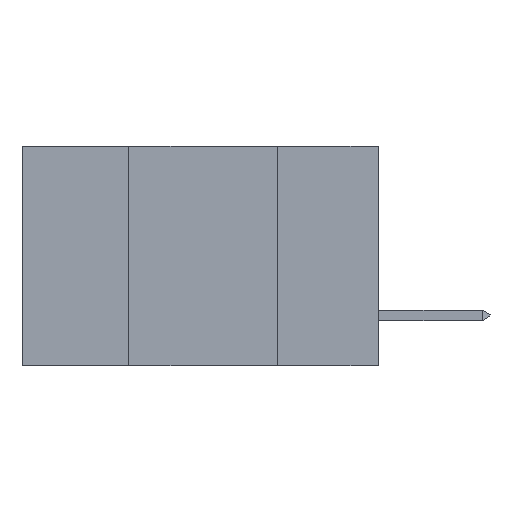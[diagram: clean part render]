
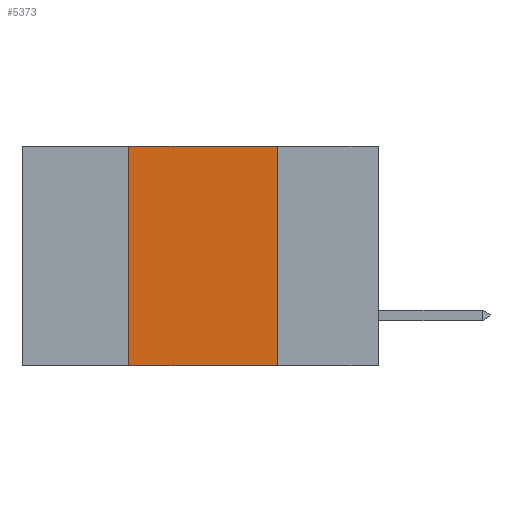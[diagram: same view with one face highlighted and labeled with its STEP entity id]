
A CAD part, left-side view. The second image highlights one B-rep face of the part: STEP entity #5373.
In plain terms, the highlighted planar face has unit normal (-1, 0, 0).
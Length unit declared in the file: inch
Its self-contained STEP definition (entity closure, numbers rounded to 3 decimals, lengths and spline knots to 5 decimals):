
#425 = VERTEX_POINT ( 'NONE', #5823 ) ;
#1154 = CARTESIAN_POINT ( 'NONE',  ( 0., 0.17, -0.37 ) ) ;
#1305 = FACE_OUTER_BOUND ( 'NONE', #10136, .T. ) ;
#1309 = LINE ( 'NONE', #15162, #5627 ) ;
#2109 = CARTESIAN_POINT ( 'NONE',  ( 0., 0.42, 0. ) ) ;
#2255 = EDGE_CURVE ( 'NONE', #4426, #10716, #3653, .T. ) ;
#2405 = CARTESIAN_POINT ( 'NONE',  ( 0., 0.6, -0.37 ) ) ;
#2849 = ORIENTED_EDGE ( 'NONE', *, *, #15964, .F. ) ;
#3488 = ORIENTED_EDGE ( 'NONE', *, *, #2255, .T. ) ;
#3515 = CARTESIAN_POINT ( 'NONE',  ( 0., 0.17, -0.37 ) ) ;
#3653 = LINE ( 'NONE', #2405, #3752 ) ;
#3752 = VECTOR ( 'NONE', #15011, 39.37008 ) ;
#3869 = CARTESIAN_POINT ( 'NONE',  ( 0., 0.6, 0. ) ) ;
#4426 = VERTEX_POINT ( 'NONE', #16137 ) ;
#5008 = LINE ( 'NONE', #1154, #6427 ) ;
#5373 = ADVANCED_FACE ( 'NONE', ( #1305 ), #12753, .F. ) ;
#5627 = VECTOR ( 'NONE', #13747, 39.37008 ) ;
#5731 = DIRECTION ( 'NONE',  ( 0., -1., 0. ) ) ;
#5823 = CARTESIAN_POINT ( 'NONE',  ( 0., 0.17, 0. ) ) ;
#6109 = EDGE_CURVE ( 'NONE', #15588, #425, #7060, .T. ) ;
#6182 = DIRECTION ( 'NONE',  ( 0., 0., -1. ) ) ;
#6353 = ORIENTED_EDGE ( 'NONE', *, *, #15987, .F. ) ;
#6425 = VECTOR ( 'NONE', #5731, 39.37008 ) ;
#6427 = VECTOR ( 'NONE', #6182, 39.37008 ) ;
#6512 = DIRECTION ( 'NONE',  ( 0., 0., -1. ) ) ;
#7060 = LINE ( 'NONE', #12317, #6425 ) ;
#7831 = DIRECTION ( 'NONE',  ( 1., 0., 0. ) ) ;
#8901 = AXIS2_PLACEMENT_3D ( 'NONE', #3869, #7831, #6512 ) ;
#9318 = ORIENTED_EDGE ( 'NONE', *, *, #6109, .F. ) ;
#10136 = EDGE_LOOP ( 'NONE', ( #2849, #9318, #6353, #3488 ) ) ;
#10716 = VERTEX_POINT ( 'NONE', #3515 ) ;
#12317 = CARTESIAN_POINT ( 'NONE',  ( 0., 0.6, 0. ) ) ;
#12753 = PLANE ( 'NONE',  #8901 ) ;
#13747 = DIRECTION ( 'NONE',  ( 0., 0., 1. ) ) ;
#15011 = DIRECTION ( 'NONE',  ( 0., -1., 0. ) ) ;
#15162 = CARTESIAN_POINT ( 'NONE',  ( 0., 0.42, -0.37 ) ) ;
#15588 = VERTEX_POINT ( 'NONE', #2109 ) ;
#15964 = EDGE_CURVE ( 'NONE', #425, #10716, #5008, .T. ) ;
#15987 = EDGE_CURVE ( 'NONE', #4426, #15588, #1309, .T. ) ;
#16137 = CARTESIAN_POINT ( 'NONE',  ( 0., 0.42, -0.37 ) ) ;
